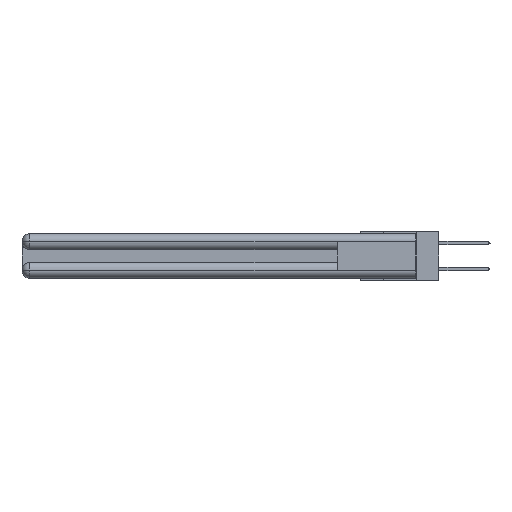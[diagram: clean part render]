
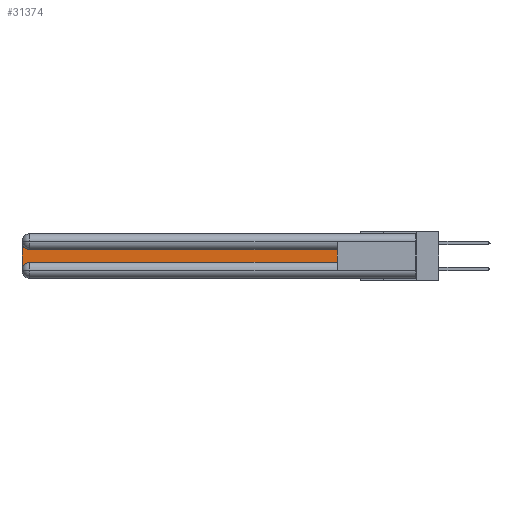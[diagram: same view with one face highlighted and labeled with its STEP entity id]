
A CAD part, left-side view. The second image highlights one B-rep face of the part: STEP entity #31374.
In plain terms, the highlighted planar face has unit normal (-1, 0, 0).
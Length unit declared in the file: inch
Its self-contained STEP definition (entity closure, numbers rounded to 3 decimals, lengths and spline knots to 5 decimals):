
#362 = EDGE_CURVE ( 'NONE', #30486, #17061, #19321, .T. ) ;
#966 = CARTESIAN_POINT ( 'NONE',  ( 0.075, 0.6, -0.2175 ) ) ;
#1319 = DIRECTION ( 'NONE',  ( 0., 0., -1. ) ) ;
#3159 = VECTOR ( 'NONE', #24224, 39.37008 ) ;
#4652 = DIRECTION ( 'NONE',  ( 0., 0., -1. ) ) ;
#5590 = AXIS2_PLACEMENT_3D ( 'NONE', #16784, #27397, #1319 ) ;
#6113 = CIRCLE ( 'NONE', #26651, 0.06 ) ;
#6671 = FACE_OUTER_BOUND ( 'NONE', #6688, .T. ) ;
#6688 = EDGE_LOOP ( 'NONE', ( #20851, #32422, #32909, #12327, #9175, #8417 ) ) ;
#8051 = DIRECTION ( 'NONE',  ( 0., 0., -1. ) ) ;
#8181 = EDGE_CURVE ( 'NONE', #31486, #16362, #18692, .T. ) ;
#8417 = ORIENTED_EDGE ( 'NONE', *, *, #9832, .T. ) ;
#9175 = ORIENTED_EDGE ( 'NONE', *, *, #8181, .T. ) ;
#9832 = EDGE_CURVE ( 'NONE', #16362, #30486, #20846, .T. ) ;
#12327 = ORIENTED_EDGE ( 'NONE', *, *, #33255, .T. ) ;
#12424 = CARTESIAN_POINT ( 'NONE',  ( 0.075, 3., -0.2775 ) ) ;
#12782 = CARTESIAN_POINT ( 'NONE',  ( 0.075, 2.94, -0.2175 ) ) ;
#13749 = VERTEX_POINT ( 'NONE', #12424 ) ;
#14253 = EDGE_CURVE ( 'NONE', #21911, #13749, #33042, .T. ) ;
#16362 = VERTEX_POINT ( 'NONE', #17726 ) ;
#16784 = CARTESIAN_POINT ( 'NONE',  ( 0.075, 3., -0.1225 ) ) ;
#17013 = CARTESIAN_POINT ( 'NONE',  ( 0.075, 0.6, -0.2175 ) ) ;
#17061 = VERTEX_POINT ( 'NONE', #20218 ) ;
#17209 = DIRECTION ( 'NONE',  ( 1., 0., 0. ) ) ;
#17726 = CARTESIAN_POINT ( 'NONE',  ( 0.075, 0.6, -0.2175 ) ) ;
#17889 = DIRECTION ( 'NONE',  ( 1., 0., 0. ) ) ;
#18692 = LINE ( 'NONE', #966, #31231 ) ;
#19008 = DIRECTION ( 'NONE',  ( 0., -1., 0. ) ) ;
#19240 = CARTESIAN_POINT ( 'NONE',  ( 0.075, 0.6, -0.1225 ) ) ;
#19321 = LINE ( 'NONE', #19430, #28638 ) ;
#19430 = CARTESIAN_POINT ( 'NONE',  ( 0.075, 0.6, -0.1225 ) ) ;
#20218 = CARTESIAN_POINT ( 'NONE',  ( 0.075, 2.94, -0.1225 ) ) ;
#20238 = CARTESIAN_POINT ( 'NONE',  ( 0.075, 2.94, -0.2775 ) ) ;
#20583 = CARTESIAN_POINT ( 'NONE',  ( 0.075, 2.94, -0.0625 ) ) ;
#20846 = LINE ( 'NONE', #17013, #26959 ) ;
#20851 = ORIENTED_EDGE ( 'NONE', *, *, #362, .T. ) ;
#21911 = VERTEX_POINT ( 'NONE', #23978 ) ;
#23700 = EDGE_CURVE ( 'NONE', #17061, #21911, #32391, .T. ) ;
#23978 = CARTESIAN_POINT ( 'NONE',  ( 0.075, 3., -0.0625 ) ) ;
#24224 = DIRECTION ( 'NONE',  ( 0., 0., -1. ) ) ;
#25243 = DIRECTION ( 'NONE',  ( 0., 0., 1. ) ) ;
#26651 = AXIS2_PLACEMENT_3D ( 'NONE', #20238, #17209, #4652 ) ;
#26959 = VECTOR ( 'NONE', #25243, 39.37008 ) ;
#27242 = DIRECTION ( 'NONE',  ( 0., 1., 0. ) ) ;
#27397 = DIRECTION ( 'NONE',  ( 1., 0., 0. ) ) ;
#28638 = VECTOR ( 'NONE', #27242, 39.37008 ) ;
#29662 = PLANE ( 'NONE',  #5590 ) ;
#29673 = CARTESIAN_POINT ( 'NONE',  ( 0.075, 3., -0.2175 ) ) ;
#30486 = VERTEX_POINT ( 'NONE', #19240 ) ;
#31231 = VECTOR ( 'NONE', #19008, 39.37008 ) ;
#31374 = ADVANCED_FACE ( 'NONE', ( #6671 ), #29662, .F. ) ;
#31486 = VERTEX_POINT ( 'NONE', #12782 ) ;
#32391 = CIRCLE ( 'NONE', #33013, 0.06 ) ;
#32422 = ORIENTED_EDGE ( 'NONE', *, *, #23700, .T. ) ;
#32909 = ORIENTED_EDGE ( 'NONE', *, *, #14253, .T. ) ;
#33013 = AXIS2_PLACEMENT_3D ( 'NONE', #20583, #17889, #8051 ) ;
#33042 = LINE ( 'NONE', #29673, #3159 ) ;
#33255 = EDGE_CURVE ( 'NONE', #13749, #31486, #6113, .T. ) ;
